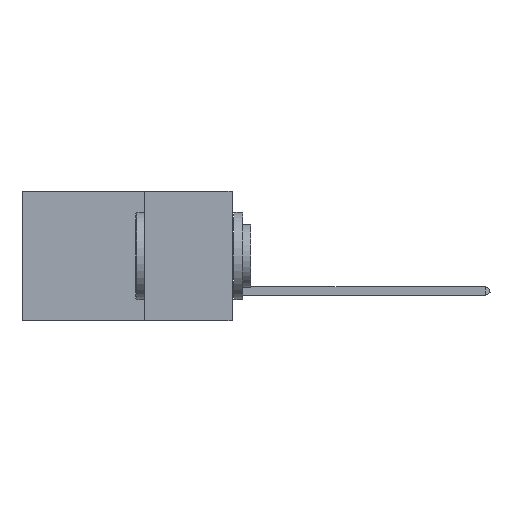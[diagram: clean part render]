
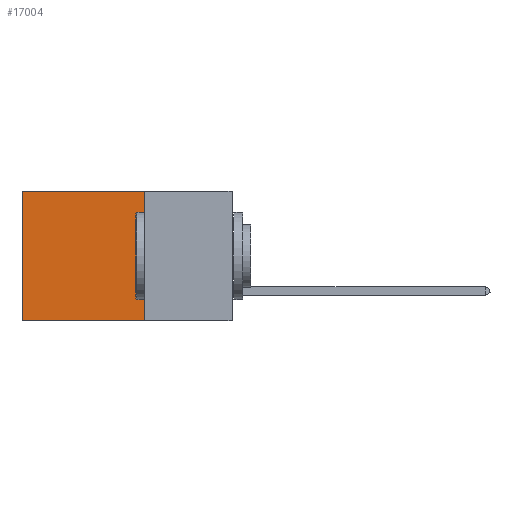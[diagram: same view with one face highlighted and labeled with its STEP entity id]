
A CAD part, left-side view. The second image highlights one B-rep face of the part: STEP entity #17004.
In plain terms, the highlighted planar face has unit normal (-1, 0, 0).
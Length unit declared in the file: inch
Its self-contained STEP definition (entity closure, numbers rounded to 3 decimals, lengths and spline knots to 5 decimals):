
#18 = VERTEX_POINT ( 'NONE', #8268 ) ;
#1096 = VECTOR ( 'NONE', #11656, 39.37008 ) ;
#1124 = EDGE_LOOP ( 'NONE', ( #3652, #14768, #16112, #15065 ) ) ;
#1514 = VECTOR ( 'NONE', #14861, 39.37008 ) ;
#2191 = VECTOR ( 'NONE', #14385, 39.37008 ) ;
#2216 = VERTEX_POINT ( 'NONE', #10578 ) ;
#2770 = AXIS2_PLACEMENT_3D ( 'NONE', #5385, #3976, #7979 ) ;
#2849 = CARTESIAN_POINT ( 'NONE',  ( 0.2875, 0.25, 0. ) ) ;
#2953 = LINE ( 'NONE', #10255, #1096 ) ;
#2969 = CARTESIAN_POINT ( 'NONE',  ( 0.2875, 0.25, -0.37 ) ) ;
#3652 = ORIENTED_EDGE ( 'NONE', *, *, #15959, .T. ) ;
#3792 = EDGE_CURVE ( 'NONE', #11223, #6997, #4664, .T. ) ;
#3976 = DIRECTION ( 'NONE',  ( 1., 0., 0. ) ) ;
#4664 = LINE ( 'NONE', #2849, #1514 ) ;
#4712 = CARTESIAN_POINT ( 'NONE',  ( 0.2875, 0.25, 0. ) ) ;
#5385 = CARTESIAN_POINT ( 'NONE',  ( 0.2875, 0.25, 0. ) ) ;
#6338 = LINE ( 'NONE', #2969, #13218 ) ;
#6795 = CARTESIAN_POINT ( 'NONE',  ( 0.2875, 0.6, 0. ) ) ;
#6997 = VERTEX_POINT ( 'NONE', #6795 ) ;
#7979 = DIRECTION ( 'NONE',  ( 0., 0., -1. ) ) ;
#8268 = CARTESIAN_POINT ( 'NONE',  ( 0.2875, 0.6, -0.37 ) ) ;
#8321 = DIRECTION ( 'NONE',  ( 0., 1., 0. ) ) ;
#8625 = LINE ( 'NONE', #4712, #2191 ) ;
#10255 = CARTESIAN_POINT ( 'NONE',  ( 0.2875, 0.6, 0. ) ) ;
#10578 = CARTESIAN_POINT ( 'NONE',  ( 0.2875, 0.25, -0.37 ) ) ;
#10779 = EDGE_CURVE ( 'NONE', #11223, #2216, #8625, .T. ) ;
#10878 = FACE_OUTER_BOUND ( 'NONE', #1124, .T. ) ;
#11156 = CARTESIAN_POINT ( 'NONE',  ( 0.2875, 0.25, 0. ) ) ;
#11223 = VERTEX_POINT ( 'NONE', #11156 ) ;
#11656 = DIRECTION ( 'NONE',  ( 0., 0., -1. ) ) ;
#13218 = VECTOR ( 'NONE', #8321, 39.37008 ) ;
#14385 = DIRECTION ( 'NONE',  ( 0., 0., -1. ) ) ;
#14768 = ORIENTED_EDGE ( 'NONE', *, *, #15512, .F. ) ;
#14861 = DIRECTION ( 'NONE',  ( 0., 1., 0. ) ) ;
#15065 = ORIENTED_EDGE ( 'NONE', *, *, #3792, .T. ) ;
#15512 = EDGE_CURVE ( 'NONE', #2216, #18, #6338, .T. ) ;
#15959 = EDGE_CURVE ( 'NONE', #6997, #18, #2953, .T. ) ;
#16112 = ORIENTED_EDGE ( 'NONE', *, *, #10779, .F. ) ;
#17004 = ADVANCED_FACE ( 'NONE', ( #10878 ), #17242, .F. ) ;
#17242 = PLANE ( 'NONE',  #2770 ) ;
